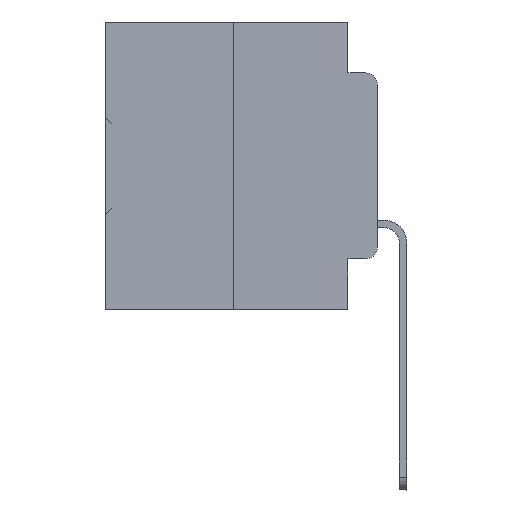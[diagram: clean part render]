
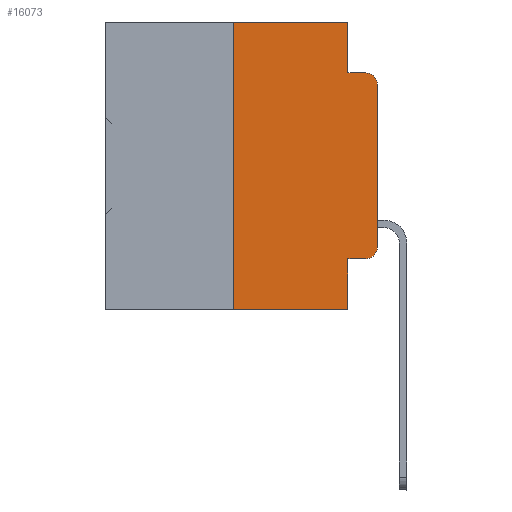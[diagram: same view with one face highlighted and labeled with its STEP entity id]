
A CAD part, left-side view. The second image highlights one B-rep face of the part: STEP entity #16073.
In plain terms, the highlighted planar face has unit normal (-1, 0, 0).
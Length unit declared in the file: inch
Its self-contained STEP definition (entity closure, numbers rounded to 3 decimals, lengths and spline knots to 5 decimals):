
#381 = VECTOR ( 'NONE', #26359, 39.37008 ) ;
#1669 = DIRECTION ( 'NONE',  ( 0., -1., 0. ) ) ;
#1703 = DIRECTION ( 'NONE',  ( 0., 0., -1. ) ) ;
#1762 = VECTOR ( 'NONE', #19903, 39.37008 ) ;
#1976 = CARTESIAN_POINT ( 'NONE',  ( 0., 0.051, 0. ) ) ;
#2555 = DIRECTION ( 'NONE',  ( 0., -1., 0. ) ) ;
#2614 = LINE ( 'NONE', #10493, #7367 ) ;
#3100 = ORIENTED_EDGE ( 'NONE', *, *, #3713, .F. ) ;
#3713 = EDGE_CURVE ( 'NONE', #28414, #31857, #20164, .T. ) ;
#4227 = DIRECTION ( 'NONE',  ( -1., 0., 0. ) ) ;
#5693 = LINE ( 'NONE', #38582, #31925 ) ;
#5708 = DIRECTION ( 'NONE',  ( 0., 0., 1. ) ) ;
#6518 = CARTESIAN_POINT ( 'NONE',  ( 0., 0.02, -0.1085 ) ) ;
#6745 = VERTEX_POINT ( 'NONE', #34203 ) ;
#7126 = VERTEX_POINT ( 'NONE', #24173 ) ;
#7367 = VECTOR ( 'NONE', #1703, 39.37008 ) ;
#7508 = ORIENTED_EDGE ( 'NONE', *, *, #12202, .F. ) ;
#7863 = CIRCLE ( 'NONE', #8905, 0.02 ) ;
#8063 = VECTOR ( 'NONE', #17203, 39.37008 ) ;
#8787 = CARTESIAN_POINT ( 'NONE',  ( 0., 0., 0. ) ) ;
#8905 = AXIS2_PLACEMENT_3D ( 'NONE', #6518, #33854, #18942 ) ;
#9345 = EDGE_LOOP ( 'NONE', ( #30230, #24838, #16857, #31849, #10172, #3100, #15938, #7508, #16062, #21000 ) ) ;
#9572 = EDGE_CURVE ( 'NONE', #7126, #13976, #14499, .T. ) ;
#9971 = VECTOR ( 'NONE', #2555, 39.37008 ) ;
#10172 = ORIENTED_EDGE ( 'NONE', *, *, #11792, .F. ) ;
#10493 = CARTESIAN_POINT ( 'NONE',  ( 0., 0.051, 0. ) ) ;
#10787 = VERTEX_POINT ( 'NONE', #21808 ) ;
#11792 = EDGE_CURVE ( 'NONE', #31857, #18274, #20924, .T. ) ;
#12024 = CARTESIAN_POINT ( 'NONE',  ( 0., 0.25, -0.5 ) ) ;
#12041 = EDGE_CURVE ( 'NONE', #17760, #7126, #27552, .T. ) ;
#12202 = EDGE_CURVE ( 'NONE', #26876, #6745, #23314, .T. ) ;
#13025 = FACE_OUTER_BOUND ( 'NONE', #9345, .T. ) ;
#13543 = VECTOR ( 'NONE', #5708, 39.37008 ) ;
#13976 = VERTEX_POINT ( 'NONE', #25088 ) ;
#14476 = PLANE ( 'NONE',  #32095 ) ;
#14499 = LINE ( 'NONE', #8787, #13543 ) ;
#15938 = ORIENTED_EDGE ( 'NONE', *, *, #20240, .T. ) ;
#16062 = ORIENTED_EDGE ( 'NONE', *, *, #26982, .T. ) ;
#16073 = ADVANCED_FACE ( 'NONE', ( #13025 ), #14476, .F. ) ;
#16552 = LINE ( 'NONE', #16848, #1762 ) ;
#16848 = CARTESIAN_POINT ( 'NONE',  ( 0., 0.473, -0.5 ) ) ;
#16857 = ORIENTED_EDGE ( 'NONE', *, *, #36983, .F. ) ;
#17006 = CARTESIAN_POINT ( 'NONE',  ( 0., 0.02, -0.4115 ) ) ;
#17203 = DIRECTION ( 'NONE',  ( 0., -1., 0. ) ) ;
#17760 = VERTEX_POINT ( 'NONE', #17006 ) ;
#18274 = VERTEX_POINT ( 'NONE', #31345 ) ;
#18942 = DIRECTION ( 'NONE',  ( 0., 0., -1. ) ) ;
#19057 = DIRECTION ( 'NONE',  ( 0., 0., -1. ) ) ;
#19903 = DIRECTION ( 'NONE',  ( 0., -1., 0. ) ) ;
#20052 = DIRECTION ( 'NONE',  ( 0., 0., 1. ) ) ;
#20164 = LINE ( 'NONE', #35254, #30605 ) ;
#20240 = EDGE_CURVE ( 'NONE', #28414, #6745, #16552, .T. ) ;
#20924 = LINE ( 'NONE', #35467, #8063 ) ;
#20945 = LINE ( 'NONE', #26404, #9971 ) ;
#21000 = ORIENTED_EDGE ( 'NONE', *, *, #12041, .T. ) ;
#21293 = EDGE_CURVE ( 'NONE', #18274, #35793, #2614, .T. ) ;
#21808 = CARTESIAN_POINT ( 'NONE',  ( 0., 0.02, -0.0885 ) ) ;
#23227 = CARTESIAN_POINT ( 'NONE',  ( 0., 0.051, -0.4115 ) ) ;
#23314 = LINE ( 'NONE', #1976, #381 ) ;
#24173 = CARTESIAN_POINT ( 'NONE',  ( 0., 0., -0.3915 ) ) ;
#24838 = ORIENTED_EDGE ( 'NONE', *, *, #32622, .T. ) ;
#25088 = CARTESIAN_POINT ( 'NONE',  ( 0., 0., -0.1085 ) ) ;
#25433 = CARTESIAN_POINT ( 'NONE',  ( 0., 0.02, -0.3915 ) ) ;
#26359 = DIRECTION ( 'NONE',  ( 0., 0., -1. ) ) ;
#26404 = CARTESIAN_POINT ( 'NONE',  ( 0., 0.051, -0.4115 ) ) ;
#26670 = DIRECTION ( 'NONE',  ( 0., 0., -1. ) ) ;
#26806 = DIRECTION ( 'NONE',  ( 1., 0., 0. ) ) ;
#26876 = VERTEX_POINT ( 'NONE', #23227 ) ;
#26982 = EDGE_CURVE ( 'NONE', #26876, #17760, #20945, .T. ) ;
#27552 = CIRCLE ( 'NONE', #31733, 0.02 ) ;
#28414 = VERTEX_POINT ( 'NONE', #12024 ) ;
#30230 = ORIENTED_EDGE ( 'NONE', *, *, #9572, .T. ) ;
#30605 = VECTOR ( 'NONE', #20052, 39.37008 ) ;
#31345 = CARTESIAN_POINT ( 'NONE',  ( 0., 0.051, 0. ) ) ;
#31733 = AXIS2_PLACEMENT_3D ( 'NONE', #25433, #4227, #19057 ) ;
#31849 = ORIENTED_EDGE ( 'NONE', *, *, #21293, .F. ) ;
#31857 = VERTEX_POINT ( 'NONE', #38587 ) ;
#31925 = VECTOR ( 'NONE', #1669, 39.37008 ) ;
#32095 = AXIS2_PLACEMENT_3D ( 'NONE', #35757, #26806, #26670 ) ;
#32622 = EDGE_CURVE ( 'NONE', #13976, #10787, #7863, .T. ) ;
#33854 = DIRECTION ( 'NONE',  ( -1., 0., 0. ) ) ;
#34203 = CARTESIAN_POINT ( 'NONE',  ( 0., 0.051, -0.5 ) ) ;
#35254 = CARTESIAN_POINT ( 'NONE',  ( 0., 0.25, 0. ) ) ;
#35467 = CARTESIAN_POINT ( 'NONE',  ( 0., 0.473, 0. ) ) ;
#35744 = CARTESIAN_POINT ( 'NONE',  ( 0., 0.051, -0.0885 ) ) ;
#35757 = CARTESIAN_POINT ( 'NONE',  ( 0., 0.473, 0. ) ) ;
#35793 = VERTEX_POINT ( 'NONE', #35744 ) ;
#36983 = EDGE_CURVE ( 'NONE', #35793, #10787, #5693, .T. ) ;
#38582 = CARTESIAN_POINT ( 'NONE',  ( 0., 0.051, -0.0885 ) ) ;
#38587 = CARTESIAN_POINT ( 'NONE',  ( 0., 0.25, 0. ) ) ;
